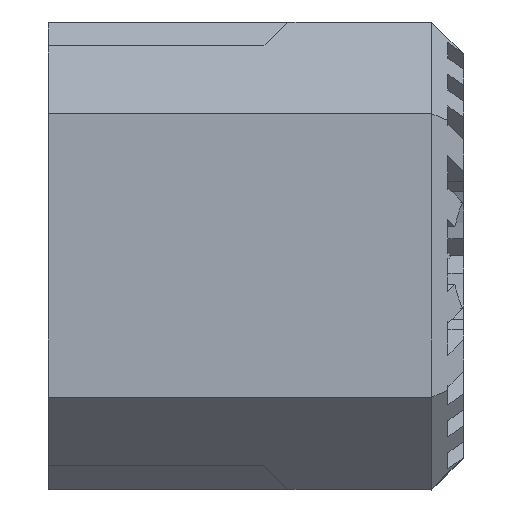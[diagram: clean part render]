
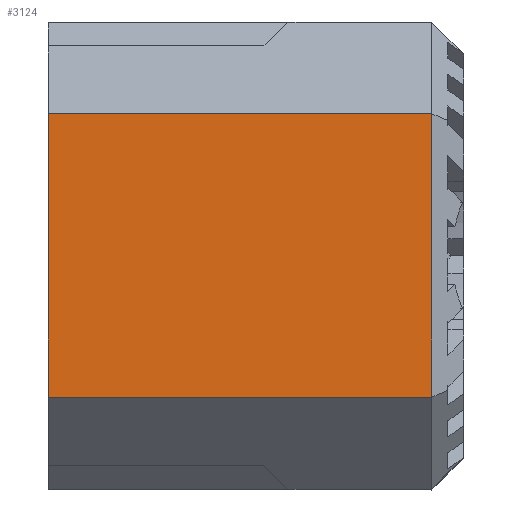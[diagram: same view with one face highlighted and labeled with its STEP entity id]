
A CAD part, top view. The second image highlights one B-rep face of the part: STEP entity #3124.
In plain terms, the highlighted planar face has unit normal (0, 0, 1).
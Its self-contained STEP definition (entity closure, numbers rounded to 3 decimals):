
#165=PLANE('',#3383);
#330=FACE_OUTER_BOUND('',#501,.T.);
#501=EDGE_LOOP('',(#2931,#2932,#2933,#2934));
#593=LINE('',#4490,#960);
#611=LINE('',#4538,#978);
#849=LINE('',#5094,#1216);
#868=LINE('',#5134,#1235);
#960=VECTOR('',#3601,10.);
#978=VECTOR('',#3647,10.);
#1216=VECTOR('',#4183,10.);
#1235=VECTOR('',#4232,10.);
#1405=VERTEX_POINT('',#4487);
#1406=VERTEX_POINT('',#4489);
#1422=VERTEX_POINT('',#4536);
#1565=VERTEX_POINT('',#4944);
#1718=EDGE_CURVE('',#1405,#1406,#593,.T.);
#1742=EDGE_CURVE('',#1422,#1405,#611,.T.);
#2022=EDGE_CURVE('',#1565,#1422,#849,.T.);
#2043=EDGE_CURVE('',#1565,#1406,#868,.T.);
#2931=ORIENTED_EDGE('',*,*,#2022,.F.);
#2932=ORIENTED_EDGE('',*,*,#2043,.T.);
#2933=ORIENTED_EDGE('',*,*,#1718,.F.);
#2934=ORIENTED_EDGE('',*,*,#1742,.F.);
#3124=ADVANCED_FACE('',(#330),#165,.T.);
#3383=AXIS2_PLACEMENT_3D('',#5139,#4240,#4241);
#3601=DIRECTION('',(0.,1.,0.));
#3647=DIRECTION('',(-1.,0.,0.));
#4183=DIRECTION('',(0.,-1.,0.));
#4232=DIRECTION('',(-1.,0.,0.));
#4240=DIRECTION('center_axis',(0.,0.,
1.));
#4241=DIRECTION('ref_axis',(0.,-1.,0.));
#4487=CARTESIAN_POINT('',(159.135,-182.355,-1.747));
#4489=CARTESIAN_POINT('',(159.135,-164.623,-1.747));
#4490=CARTESIAN_POINT('',(159.135,-165.876,-1.747));
#4536=CARTESIAN_POINT('',(183.135,-182.355,-1.747));
#4538=CARTESIAN_POINT('',(27.255,-182.355,-1.747));
#4944=CARTESIAN_POINT('',(183.135,-164.623,-1.747));
#5094=CARTESIAN_POINT('',(183.135,-172.434,-1.747));
#5134=CARTESIAN_POINT('',(164.135,-164.623,-1.747));
#5139=CARTESIAN_POINT('Origin',(-43.625,-158.264,-1.747));
